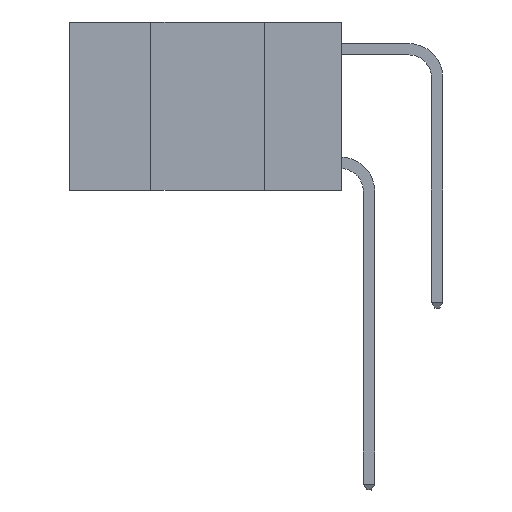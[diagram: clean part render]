
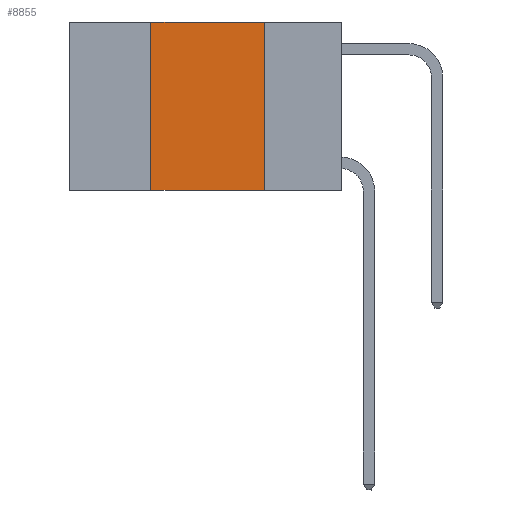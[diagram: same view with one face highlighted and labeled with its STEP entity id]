
A CAD part, left-side view. The second image highlights one B-rep face of the part: STEP entity #8855.
In plain terms, the highlighted planar face has unit normal (-1, 0, 0).
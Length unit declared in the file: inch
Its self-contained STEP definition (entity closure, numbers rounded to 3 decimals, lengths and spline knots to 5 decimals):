
#192 = CARTESIAN_POINT ( 'NONE',  ( 0., 0.17, 0. ) ) ;
#235 = EDGE_CURVE ( 'NONE', #3982, #9561, #4787, .T. ) ;
#946 = EDGE_LOOP ( 'NONE', ( #9882, #4968, #8602, #11630 ) ) ;
#2115 = DIRECTION ( 'NONE',  ( 1., 0., 0. ) ) ;
#2751 = DIRECTION ( 'NONE',  ( 0., -1., 0. ) ) ;
#3982 = VERTEX_POINT ( 'NONE', #15041 ) ;
#4558 = VERTEX_POINT ( 'NONE', #8375 ) ;
#4787 = LINE ( 'NONE', #7243, #8056 ) ;
#4968 = ORIENTED_EDGE ( 'NONE', *, *, #235, .F. ) ;
#6803 = CARTESIAN_POINT ( 'NONE',  ( 0., 0.17, -0.37 ) ) ;
#6839 = VECTOR ( 'NONE', #10049, 39.37008 ) ;
#6938 = VERTEX_POINT ( 'NONE', #6803 ) ;
#7009 = DIRECTION ( 'NONE',  ( 0., 0., 1. ) ) ;
#7214 = LINE ( 'NONE', #192, #6839 ) ;
#7243 = CARTESIAN_POINT ( 'NONE',  ( 0., 0.6, 0. ) ) ;
#7550 = EDGE_CURVE ( 'NONE', #4558, #3982, #14571, .T. ) ;
#8056 = VECTOR ( 'NONE', #11012, 39.37008 ) ;
#8202 = VECTOR ( 'NONE', #7009, 39.37008 ) ;
#8348 = EDGE_CURVE ( 'NONE', #4558, #6938, #11596, .T. ) ;
#8375 = CARTESIAN_POINT ( 'NONE',  ( 0., 0.42, -0.37 ) ) ;
#8602 = ORIENTED_EDGE ( 'NONE', *, *, #7550, .F. ) ;
#8855 = ADVANCED_FACE ( 'NONE', ( #11485 ), #9507, .F. ) ;
#8918 = CARTESIAN_POINT ( 'NONE',  ( 0., 0.6, -0.37 ) ) ;
#9507 = PLANE ( 'NONE',  #10257 ) ;
#9561 = VERTEX_POINT ( 'NONE', #14508 ) ;
#9882 = ORIENTED_EDGE ( 'NONE', *, *, #13191, .F. ) ;
#10049 = DIRECTION ( 'NONE',  ( 0., 0., -1. ) ) ;
#10257 = AXIS2_PLACEMENT_3D ( 'NONE', #13944, #2115, #10636 ) ;
#10551 = VECTOR ( 'NONE', #2751, 39.37008 ) ;
#10636 = DIRECTION ( 'NONE',  ( 0., 0., -1. ) ) ;
#11012 = DIRECTION ( 'NONE',  ( 0., -1., 0. ) ) ;
#11485 = FACE_OUTER_BOUND ( 'NONE', #946, .T. ) ;
#11596 = LINE ( 'NONE', #8918, #10551 ) ;
#11630 = ORIENTED_EDGE ( 'NONE', *, *, #8348, .T. ) ;
#12714 = CARTESIAN_POINT ( 'NONE',  ( 0., 0.42, 0. ) ) ;
#13191 = EDGE_CURVE ( 'NONE', #9561, #6938, #7214, .T. ) ;
#13944 = CARTESIAN_POINT ( 'NONE',  ( 0., 0.6, 0. ) ) ;
#14508 = CARTESIAN_POINT ( 'NONE',  ( 0., 0.17, 0. ) ) ;
#14571 = LINE ( 'NONE', #12714, #8202 ) ;
#15041 = CARTESIAN_POINT ( 'NONE',  ( 0., 0.42, 0. ) ) ;
